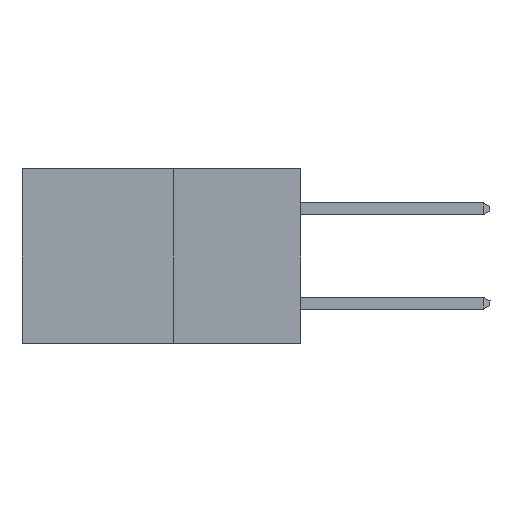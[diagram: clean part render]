
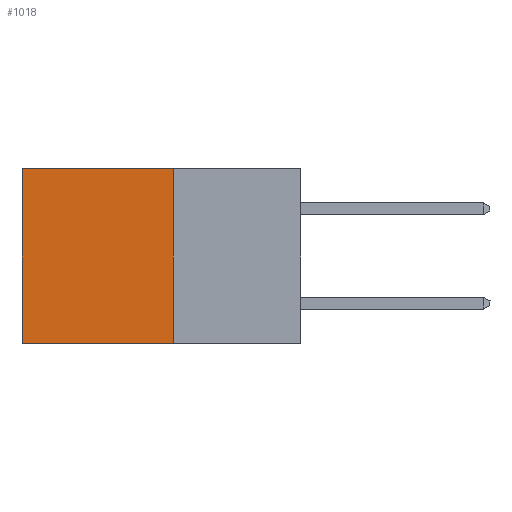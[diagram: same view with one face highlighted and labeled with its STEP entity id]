
A CAD part, left-side view. The second image highlights one B-rep face of the part: STEP entity #1018.
In plain terms, the highlighted planar face has unit normal (-1, 0, 0).
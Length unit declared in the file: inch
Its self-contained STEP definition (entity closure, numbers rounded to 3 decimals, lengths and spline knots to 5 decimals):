
#206 = AXIS2_PLACEMENT_3D ( 'NONE', #2472, #475, #313 ) ;
#313 = DIRECTION ( 'NONE',  ( 0., 0., -1. ) ) ;
#384 = LINE ( 'NONE', #6999, #8558 ) ;
#475 = DIRECTION ( 'NONE',  ( 1., 0., 0. ) ) ;
#718 = ORIENTED_EDGE ( 'NONE', *, *, #8667, .F. ) ;
#881 = LINE ( 'NONE', #4801, #6767 ) ;
#1018 = ADVANCED_FACE ( 'NONE', ( #7635 ), #5397, .F. ) ;
#1229 = EDGE_CURVE ( 'NONE', #3366, #8148, #8780, .T. ) ;
#1821 = DIRECTION ( 'NONE',  ( 0., 1., 0. ) ) ;
#2226 = EDGE_CURVE ( 'NONE', #6844, #3366, #8293, .T. ) ;
#2472 = CARTESIAN_POINT ( 'NONE',  ( 0.277, 0.27, -0.37 ) ) ;
#2877 = VERTEX_POINT ( 'NONE', #3015 ) ;
#3015 = CARTESIAN_POINT ( 'NONE',  ( 0.277, 0.27, -0.37 ) ) ;
#3366 = VERTEX_POINT ( 'NONE', #4457 ) ;
#4168 = VECTOR ( 'NONE', #1821, 39.37008 ) ;
#4457 = CARTESIAN_POINT ( 'NONE',  ( 0.277, 0.59, 0. ) ) ;
#4711 = VECTOR ( 'NONE', #9701, 39.37008 ) ;
#4801 = CARTESIAN_POINT ( 'NONE',  ( 0.277, 0.27, -0.37 ) ) ;
#4842 = DIRECTION ( 'NONE',  ( 0., 1., 0. ) ) ;
#5397 = PLANE ( 'NONE',  #206 ) ;
#6300 = EDGE_LOOP ( 'NONE', ( #7121, #9022, #718, #7335 ) ) ;
#6321 = CARTESIAN_POINT ( 'NONE',  ( 0.277, 0.27, 0. ) ) ;
#6767 = VECTOR ( 'NONE', #4842, 39.37008 ) ;
#6844 = VERTEX_POINT ( 'NONE', #6321 ) ;
#6884 = DIRECTION ( 'NONE',  ( 0., 0., -1. ) ) ;
#6999 = CARTESIAN_POINT ( 'NONE',  ( 0.277, 0.27, -0.37 ) ) ;
#7014 = EDGE_CURVE ( 'NONE', #2877, #8148, #881, .T. ) ;
#7121 = ORIENTED_EDGE ( 'NONE', *, *, #1229, .T. ) ;
#7335 = ORIENTED_EDGE ( 'NONE', *, *, #2226, .T. ) ;
#7550 = CARTESIAN_POINT ( 'NONE',  ( 0.277, 0.27, 0. ) ) ;
#7635 = FACE_OUTER_BOUND ( 'NONE', #6300, .T. ) ;
#7697 = CARTESIAN_POINT ( 'NONE',  ( 0.277, 0.59, -0.37 ) ) ;
#8148 = VERTEX_POINT ( 'NONE', #9305 ) ;
#8293 = LINE ( 'NONE', #7550, #4168 ) ;
#8558 = VECTOR ( 'NONE', #6884, 39.37008 ) ;
#8667 = EDGE_CURVE ( 'NONE', #6844, #2877, #384, .T. ) ;
#8780 = LINE ( 'NONE', #7697, #4711 ) ;
#9022 = ORIENTED_EDGE ( 'NONE', *, *, #7014, .F. ) ;
#9305 = CARTESIAN_POINT ( 'NONE',  ( 0.277, 0.59, -0.37 ) ) ;
#9701 = DIRECTION ( 'NONE',  ( 0., 0., -1. ) ) ;
